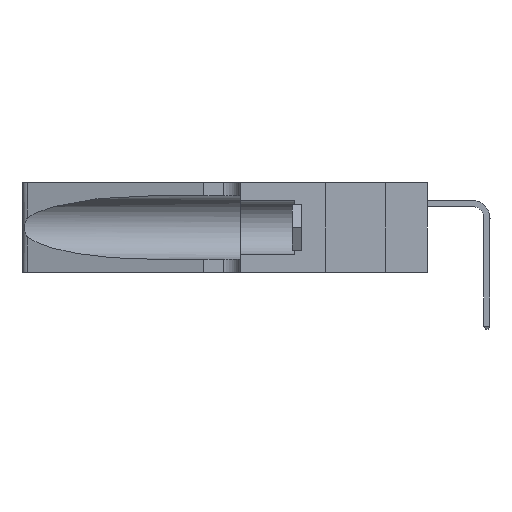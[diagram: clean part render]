
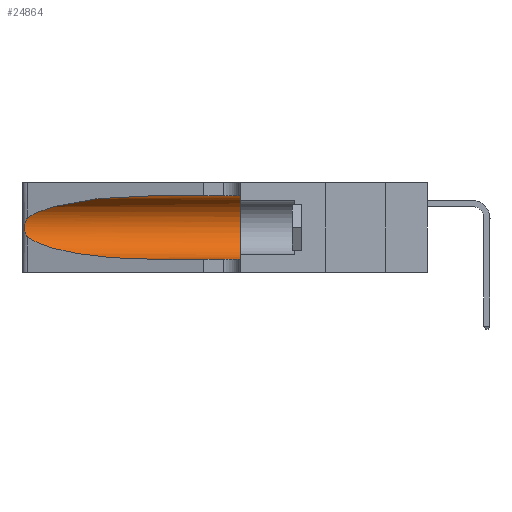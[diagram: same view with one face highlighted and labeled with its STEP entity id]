
A CAD part, left-side view. The second image highlights one B-rep face of the part: STEP entity #24864.
In plain terms, the highlighted cylindrical face has radius 3.308 mm (diameter 6.617 mm), a partial arc.
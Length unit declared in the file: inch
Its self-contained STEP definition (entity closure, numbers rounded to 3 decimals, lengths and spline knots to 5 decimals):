
#701 = DIRECTION ( 'NONE',  ( 0., 0., 1. ) ) ;
#1455 = CARTESIAN_POINT ( 'NONE',  ( 0.1305, 0.35, 0.05475 ) ) ;
#1669 = CARTESIAN_POINT ( 'NONE',  ( 0.18966, 0.96281, 0.31525 ) ) ;
#1873 = CARTESIAN_POINT ( 'NONE',  ( 0.25555, 1.22994, 0.2215 ) ) ;
#4852 = EDGE_CURVE ( 'NONE', #16553, #18891, #12918, .T. ) ;
#5555 = CARTESIAN_POINT ( 'NONE',  ( 0.2373, 1.15595, 0.28018 ) ) ;
#5757 = CARTESIAN_POINT ( 'NONE',  ( 0.25787, 1.23484, 0.2124 ) ) ;
#5803 = CARTESIAN_POINT ( 'NONE',  ( 0.25487, 1.22718, 0.14631 ) ) ;
#5990 = AXIS2_PLACEMENT_3D ( 'NONE', #46408, #23548, #701 ) ;
#6501 = DIRECTION ( 'NONE',  ( 0., -1., 0. ) ) ;
#7482 = CARTESIAN_POINT ( 'NONE',  ( 0.1305, 0.72297, 0.05475 ) ) ;
#8750 = LINE ( 'NONE', #17810, #16446 ) ;
#9581 = CARTESIAN_POINT ( 'NONE',  ( 0.26018, 1.23835, 0.19895 ) ) ;
#9917 = LINE ( 'NONE', #13257, #11094 ) ;
#11094 = VECTOR ( 'NONE', #24755, 39.37008 ) ;
#12918 = B_SPLINE_CURVE_WITH_KNOTS ( 'NONE', 3,
 ( #28610, #1873, #47574, #5757, #32392, #9581, #36243, #13388, #40072, #17215, #43908, #21027, #47736, #24897 ),
 .UNSPECIFIED., .F., .F.,
 ( 4, 2, 2, 2, 2, 2, 4 ),
 ( 0., 0.00027, 0.00053, 0.00107, 0.0016, 0.00187, 0.00214 ),
 .UNSPECIFIED. ) ;
#13257 = CARTESIAN_POINT ( 'NONE',  ( 0.1305, 1.61858, 0.31525 ) ) ;
#13388 = CARTESIAN_POINT ( 'NONE',  ( 0.26075, 1.23896, 0.178 ) ) ;
#14156 = CARTESIAN_POINT ( 'NONE',  ( 0.1305, 1.61858, 0.185 ) ) ;
#14734 = EDGE_CURVE ( 'NONE', #44806, #24072, #9917, .T. ) ;
#15330 = CARTESIAN_POINT ( 'NONE',  ( 0.1305, 0.72297, 0.31525 ) ) ;
#16446 = VECTOR ( 'NONE', #6501, 39.37008 ) ;
#16553 = VERTEX_POINT ( 'NONE', #39288 ) ;
#17215 = CARTESIAN_POINT ( 'NONE',  ( 0.25856, 1.23593, 0.16098 ) ) ;
#17810 = CARTESIAN_POINT ( 'NONE',  ( 0.1305, 1.61858, 0.05475 ) ) ;
#17964 = DIRECTION ( 'NONE',  ( 0., 0., -1. ) ) ;
#18665 = ORIENTED_EDGE ( 'NONE', *, *, #39269, .T. ) ;
#18891 = VERTEX_POINT ( 'NONE', #5803 ) ;
#20667 = CARTESIAN_POINT ( 'NONE',  ( 0.1305, 0.72297, 0.31525 ) ) ;
#21027 = CARTESIAN_POINT ( 'NONE',  ( 0.25639, 1.23186, 0.15144 ) ) ;
#21029 = EDGE_CURVE ( 'NONE', #18891, #41808, #43055, .T. ) ;
#21038 = ORIENTED_EDGE ( 'NONE', *, *, #4852, .T. ) ;
#22624 = CARTESIAN_POINT ( 'NONE',  ( 0.2373, 1.15595, 0.08982 ) ) ;
#23548 = DIRECTION ( 'NONE',  ( 0., 1., 0. ) ) ;
#24072 = VERTEX_POINT ( 'NONE', #24373 ) ;
#24373 = CARTESIAN_POINT ( 'NONE',  ( 0.1305, 0.35, 0.31525 ) ) ;
#24755 = DIRECTION ( 'NONE',  ( 0., -1., 0. ) ) ;
#24864 = ADVANCED_FACE ( 'NONE', ( #26133 ), #24924, .F. ) ;
#24897 = CARTESIAN_POINT ( 'NONE',  ( 0.25487, 1.22718, 0.14631 ) ) ;
#24924 = CYLINDRICAL_SURFACE ( 'NONE', #26704, 0.13025 ) ;
#25800 = EDGE_CURVE ( 'NONE', #24072, #32866, #42189, .T. ) ;
#26133 = FACE_OUTER_BOUND ( 'NONE', #28393, .T. ) ;
#26581 = EDGE_CURVE ( 'NONE', #41808, #32866, #8750, .T. ) ;
#26704 = AXIS2_PLACEMENT_3D ( 'NONE', #14156, #48326, #17964 ) ;
#28393 = EDGE_LOOP ( 'NONE', ( #18665, #21038, #34251, #29499, #39640, #41620 ) ) ;
#28610 = CARTESIAN_POINT ( 'NONE',  ( 0.25487, 1.22718, 0.22369 ) ) ;
#29499 = ORIENTED_EDGE ( 'NONE', *, *, #26581, .T. ) ;
#30310 = CARTESIAN_POINT ( 'NONE',  ( 0.18966, 0.96281, 0.05475 ) ) ;
#32194 = CARTESIAN_POINT ( 'NONE',  ( 0.25487, 1.22718, 0.22369 ) ) ;
#32392 = CARTESIAN_POINT ( 'NONE',  ( 0.25854, 1.2359, 0.20912 ) ) ;
#32866 = VERTEX_POINT ( 'NONE', #1455 ) ;
#34251 = ORIENTED_EDGE ( 'NONE', *, *, #21029, .T. ) ;
#35501 = CARTESIAN_POINT ( 'NONE',  ( 0.1305, 0.72297, 0.05475 ) ) ;
#36243 = CARTESIAN_POINT ( 'NONE',  ( 0.26075, 1.23896, 0.19203 ) ) ;
#39269 = EDGE_CURVE ( 'NONE', #44806, #16553, #39411, .T. ) ;
#39288 = CARTESIAN_POINT ( 'NONE',  ( 0.25487, 1.22718, 0.22369 ) ) ;
#39411 =( BOUNDED_CURVE ( )  B_SPLINE_CURVE ( 3, ( #20667, #1669, #5555, #32194 ),
 .UNSPECIFIED., .F., .F. ) 
 B_SPLINE_CURVE_WITH_KNOTS ( ( 4, 4 ),
 ( 1.5708, 2.84003 ),
 .UNSPECIFIED. ) 
 CURVE ( )  GEOMETRIC_REPRESENTATION_ITEM ( )  RATIONAL_B_SPLINE_CURVE ( ( 1., 0.87, 0.87, 1. ) ) 
 REPRESENTATION_ITEM ( '' )  );
#39640 = ORIENTED_EDGE ( 'NONE', *, *, #25800, .F. ) ;
#40072 = CARTESIAN_POINT ( 'NONE',  ( 0.26017, 1.23833, 0.17102 ) ) ;
#41620 = ORIENTED_EDGE ( 'NONE', *, *, #14734, .F. ) ;
#41808 = VERTEX_POINT ( 'NONE', #35501 ) ;
#42189 = CIRCLE ( 'NONE', #5990, 0.13025 ) ;
#43055 =( BOUNDED_CURVE ( )  B_SPLINE_CURVE ( 3, ( #49288, #22624, #30310, #7482 ),
 .UNSPECIFIED., .F., .T. ) 
 B_SPLINE_CURVE_WITH_KNOTS ( ( 4, 4 ),
 ( 3.44316, 4.71239 ),
 .UNSPECIFIED. ) 
 CURVE ( )  GEOMETRIC_REPRESENTATION_ITEM ( )  RATIONAL_B_SPLINE_CURVE ( ( 1., 0.87, 0.87, 1. ) ) 
 REPRESENTATION_ITEM ( '' )  );
#43908 = CARTESIAN_POINT ( 'NONE',  ( 0.25789, 1.23486, 0.15765 ) ) ;
#44806 = VERTEX_POINT ( 'NONE', #15330 ) ;
#46408 = CARTESIAN_POINT ( 'NONE',  ( 0.1305, 0.35, 0.185 ) ) ;
#47574 = CARTESIAN_POINT ( 'NONE',  ( 0.25639, 1.23184, 0.21858 ) ) ;
#47736 = CARTESIAN_POINT ( 'NONE',  ( 0.25555, 1.22993, 0.14849 ) ) ;
#48326 = DIRECTION ( 'NONE',  ( 0., -1., 0. ) ) ;
#49288 = CARTESIAN_POINT ( 'NONE',  ( 0.25487, 1.22718, 0.14631 ) ) ;
